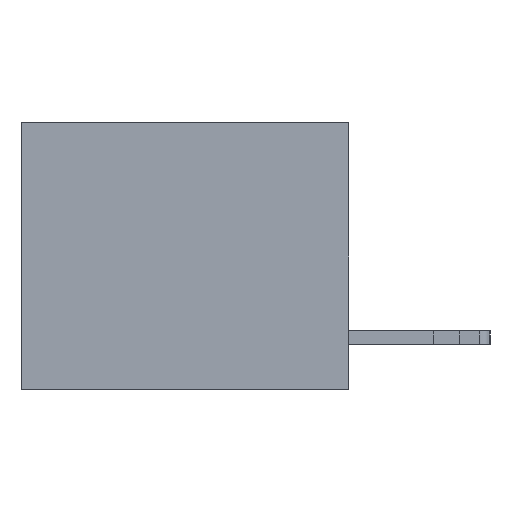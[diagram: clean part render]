
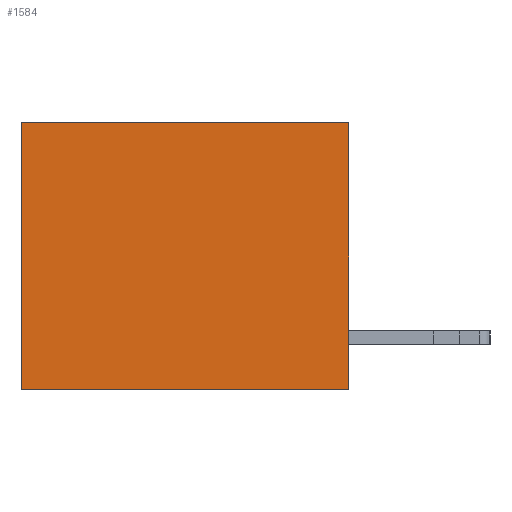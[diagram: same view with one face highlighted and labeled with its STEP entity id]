
A CAD part, left-side view. The second image highlights one B-rep face of the part: STEP entity #1584.
In plain terms, the highlighted planar face has unit normal (-1, 0, 0).
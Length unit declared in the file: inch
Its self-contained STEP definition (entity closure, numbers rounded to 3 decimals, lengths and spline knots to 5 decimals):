
#229 = VERTEX_POINT ( 'NONE', #23411 ) ;
#688 = CARTESIAN_POINT ( 'NONE',  ( 0.3165, 0., -0.49 ) ) ;
#1584 = ADVANCED_FACE ( 'NONE', ( #9725 ), #22497, .F. ) ;
#1619 = CARTESIAN_POINT ( 'NONE',  ( 0.3165, 0.6, 0. ) ) ;
#4008 = CARTESIAN_POINT ( 'NONE',  ( 0.3165, 0., -0.49 ) ) ;
#4046 = VERTEX_POINT ( 'NONE', #1619 ) ;
#5701 = VERTEX_POINT ( 'NONE', #16297 ) ;
#5849 = CARTESIAN_POINT ( 'NONE',  ( 0.3165, 0., -0.49 ) ) ;
#5944 = DIRECTION ( 'NONE',  ( 0., 0., -1. ) ) ;
#6829 = VERTEX_POINT ( 'NONE', #9837 ) ;
#7392 = ORIENTED_EDGE ( 'NONE', *, *, #11978, .F. ) ;
#7421 = EDGE_CURVE ( 'NONE', #4046, #229, #17592, .T. ) ;
#9725 = FACE_OUTER_BOUND ( 'NONE', #12901, .T. ) ;
#9837 = CARTESIAN_POINT ( 'NONE',  ( 0.3165, 0., 0. ) ) ;
#11745 = DIRECTION ( 'NONE',  ( 0., 0., -1. ) ) ;
#11978 = EDGE_CURVE ( 'NONE', #5701, #229, #15317, .T. ) ;
#12901 = EDGE_LOOP ( 'NONE', ( #16692, #7392, #13289, #19474 ) ) ;
#13029 = VECTOR ( 'NONE', #15993, 39.37008 ) ;
#13289 = ORIENTED_EDGE ( 'NONE', *, *, #13592, .F. ) ;
#13528 = DIRECTION ( 'NONE',  ( 1., 0., 0. ) ) ;
#13592 = EDGE_CURVE ( 'NONE', #6829, #5701, #19529, .T. ) ;
#13779 = AXIS2_PLACEMENT_3D ( 'NONE', #688, #13528, #18737 ) ;
#14152 = VECTOR ( 'NONE', #11745, 39.37008 ) ;
#14971 = CARTESIAN_POINT ( 'NONE',  ( 0.3165, 0.6, -0.49 ) ) ;
#15317 = LINE ( 'NONE', #4008, #18992 ) ;
#15993 = DIRECTION ( 'NONE',  ( 0., 1., 0. ) ) ;
#16230 = CARTESIAN_POINT ( 'NONE',  ( 0.3165, 0., 0. ) ) ;
#16297 = CARTESIAN_POINT ( 'NONE',  ( 0.3165, 0., -0.49 ) ) ;
#16642 = DIRECTION ( 'NONE',  ( 0., 1., 0. ) ) ;
#16692 = ORIENTED_EDGE ( 'NONE', *, *, #7421, .T. ) ;
#17592 = LINE ( 'NONE', #14971, #21285 ) ;
#18737 = DIRECTION ( 'NONE',  ( 0., 0., -1. ) ) ;
#18992 = VECTOR ( 'NONE', #16642, 39.37008 ) ;
#19474 = ORIENTED_EDGE ( 'NONE', *, *, #22194, .T. ) ;
#19529 = LINE ( 'NONE', #5849, #14152 ) ;
#21285 = VECTOR ( 'NONE', #5944, 39.37008 ) ;
#22194 = EDGE_CURVE ( 'NONE', #6829, #4046, #22877, .T. ) ;
#22497 = PLANE ( 'NONE',  #13779 ) ;
#22877 = LINE ( 'NONE', #16230, #13029 ) ;
#23411 = CARTESIAN_POINT ( 'NONE',  ( 0.3165, 0.6, -0.49 ) ) ;
